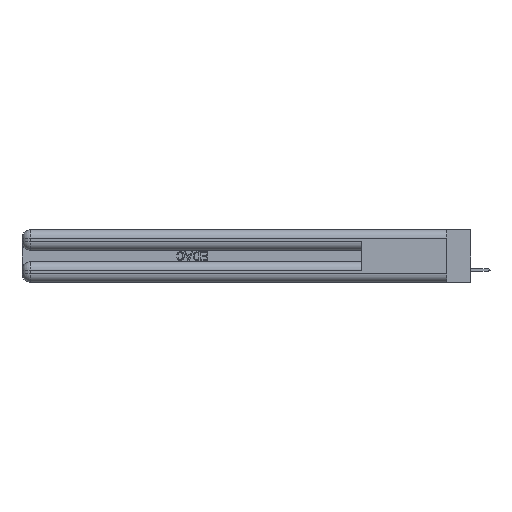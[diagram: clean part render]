
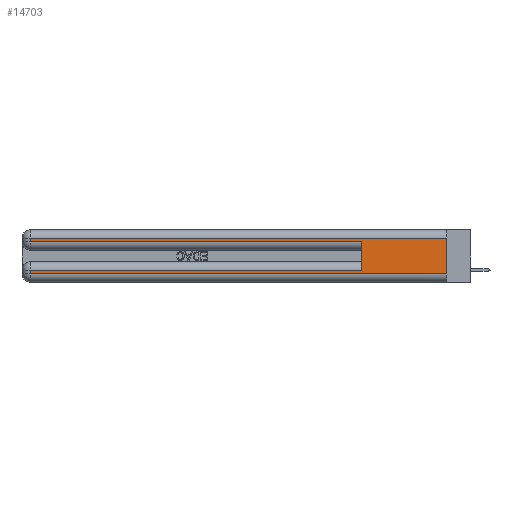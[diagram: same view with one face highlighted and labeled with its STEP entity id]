
A CAD part, left-side view. The second image highlights one B-rep face of the part: STEP entity #14703.
In plain terms, the highlighted planar face has unit normal (-1, 0, 0).
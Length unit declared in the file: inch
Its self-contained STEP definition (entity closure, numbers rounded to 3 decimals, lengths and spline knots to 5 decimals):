
#31 = LINE ( 'NONE', #12646, #24525 ) ;
#243 = ORIENTED_EDGE ( 'NONE', *, *, #22002, .F. ) ;
#800 = ORIENTED_EDGE ( 'NONE', *, *, #49027, .T. ) ;
#1507 = CARTESIAN_POINT ( 'NONE',  ( 0., 0.6, 0.145 ) ) ;
#1602 = VERTEX_POINT ( 'NONE', #45946 ) ;
#2085 = LINE ( 'NONE', #5874, #20479 ) ;
#2495 = VECTOR ( 'NONE', #20491, 39.37008 ) ;
#2865 = VERTEX_POINT ( 'NONE', #30288 ) ;
#3194 = LINE ( 'NONE', #46160, #45488 ) ;
#5763 = VERTEX_POINT ( 'NONE', #37018 ) ;
#5874 = CARTESIAN_POINT ( 'NONE',  ( 0., 0., 0.31 ) ) ;
#7429 = DIRECTION ( 'NONE',  ( 0., 1., 0. ) ) ;
#8382 = DIRECTION ( 'NONE',  ( 0., 0., -1. ) ) ;
#8921 = EDGE_LOOP ( 'NONE', ( #42582, #17783, #30205, #800, #243, #11254, #41457, #47266 ) ) ;
#9819 = VERTEX_POINT ( 'NONE', #28238 ) ;
#9856 = CARTESIAN_POINT ( 'NONE',  ( 0., 0., 0.285 ) ) ;
#10382 = DIRECTION ( 'NONE',  ( 0., -1., 0. ) ) ;
#11254 = ORIENTED_EDGE ( 'NONE', *, *, #30533, .T. ) ;
#11566 = DIRECTION ( 'NONE',  ( 0., 0., -1. ) ) ;
#12178 = DIRECTION ( 'NONE',  ( 1., 0., 0. ) ) ;
#12564 = EDGE_CURVE ( 'NONE', #5763, #39267, #20383, .T. ) ;
#12646 = CARTESIAN_POINT ( 'NONE',  ( 0., 2.94, 0.37 ) ) ;
#14016 = VECTOR ( 'NONE', #18722, 39.37008 ) ;
#14039 = AXIS2_PLACEMENT_3D ( 'NONE', #19778, #12178, #8382 ) ;
#14703 = ADVANCED_FACE ( 'NONE', ( #23076 ), #42315, .F. ) ;
#17783 = ORIENTED_EDGE ( 'NONE', *, *, #35418, .T. ) ;
#18556 = CARTESIAN_POINT ( 'NONE',  ( 0., 0., 0.31 ) ) ;
#18564 = LINE ( 'NONE', #42090, #25962 ) ;
#18722 = DIRECTION ( 'NONE',  ( 0., -1., 0. ) ) ;
#19778 = CARTESIAN_POINT ( 'NONE',  ( 0., 0., 0.37 ) ) ;
#20383 = LINE ( 'NONE', #49808, #14016 ) ;
#20479 = VECTOR ( 'NONE', #33962, 39.37008 ) ;
#20491 = DIRECTION ( 'NONE',  ( 0., 0., 1. ) ) ;
#22002 = EDGE_CURVE ( 'NONE', #9819, #2865, #46301, .T. ) ;
#23076 = FACE_OUTER_BOUND ( 'NONE', #8921, .T. ) ;
#23453 = LINE ( 'NONE', #45724, #36912 ) ;
#23971 = VERTEX_POINT ( 'NONE', #26469 ) ;
#24525 = VECTOR ( 'NONE', #42538, 39.37008 ) ;
#24837 = CARTESIAN_POINT ( 'NONE',  ( 0., 0., 0.06 ) ) ;
#25962 = VECTOR ( 'NONE', #7429, 39.37008 ) ;
#26469 = CARTESIAN_POINT ( 'NONE',  ( 0., 2.94, 0.085 ) ) ;
#28238 = CARTESIAN_POINT ( 'NONE',  ( 0., 0.6, 0.085 ) ) ;
#28831 = VERTEX_POINT ( 'NONE', #18556 ) ;
#30118 = LINE ( 'NONE', #9856, #33540 ) ;
#30205 = ORIENTED_EDGE ( 'NONE', *, *, #47158, .T. ) ;
#30288 = CARTESIAN_POINT ( 'NONE',  ( 0., 0.6, 0.285 ) ) ;
#30533 = EDGE_CURVE ( 'NONE', #9819, #23971, #18564, .T. ) ;
#33540 = VECTOR ( 'NONE', #10382, 39.37008 ) ;
#33962 = DIRECTION ( 'NONE',  ( 0., 1., 0. ) ) ;
#35418 = EDGE_CURVE ( 'NONE', #28831, #38491, #2085, .T. ) ;
#36912 = VECTOR ( 'NONE', #11566, 39.37008 ) ;
#37018 = CARTESIAN_POINT ( 'NONE',  ( 0., 2.94, 0.06 ) ) ;
#38491 = VERTEX_POINT ( 'NONE', #40184 ) ;
#38736 = EDGE_CURVE ( 'NONE', #28831, #39267, #23453, .T. ) ;
#39267 = VERTEX_POINT ( 'NONE', #24837 ) ;
#39569 = DIRECTION ( 'NONE',  ( 0., 0., -1. ) ) ;
#40184 = CARTESIAN_POINT ( 'NONE',  ( 0., 2.94, 0.31 ) ) ;
#41457 = ORIENTED_EDGE ( 'NONE', *, *, #46911, .T. ) ;
#42090 = CARTESIAN_POINT ( 'NONE',  ( 0., 0., 0.085 ) ) ;
#42315 = PLANE ( 'NONE',  #14039 ) ;
#42538 = DIRECTION ( 'NONE',  ( 0., 0., -1. ) ) ;
#42582 = ORIENTED_EDGE ( 'NONE', *, *, #38736, .F. ) ;
#45488 = VECTOR ( 'NONE', #39569, 39.37008 ) ;
#45724 = CARTESIAN_POINT ( 'NONE',  ( 0., 0., 0.37 ) ) ;
#45946 = CARTESIAN_POINT ( 'NONE',  ( 0., 2.94, 0.285 ) ) ;
#46160 = CARTESIAN_POINT ( 'NONE',  ( 0., 2.94, 0.37 ) ) ;
#46301 = LINE ( 'NONE', #1507, #2495 ) ;
#46911 = EDGE_CURVE ( 'NONE', #23971, #5763, #3194, .T. ) ;
#47158 = EDGE_CURVE ( 'NONE', #38491, #1602, #31, .T. ) ;
#47266 = ORIENTED_EDGE ( 'NONE', *, *, #12564, .T. ) ;
#49027 = EDGE_CURVE ( 'NONE', #1602, #2865, #30118, .T. ) ;
#49808 = CARTESIAN_POINT ( 'NONE',  ( 0., 0., 0.06 ) ) ;
